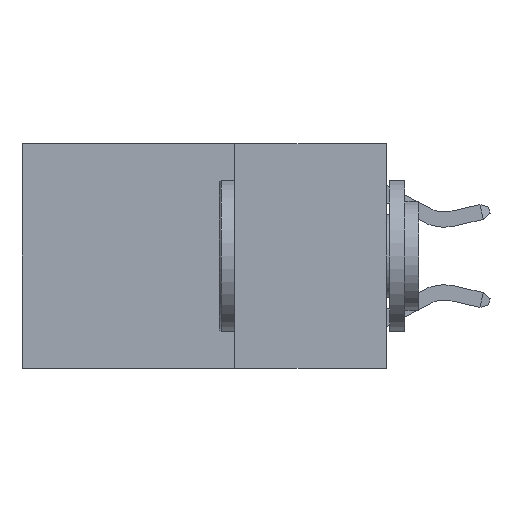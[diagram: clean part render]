
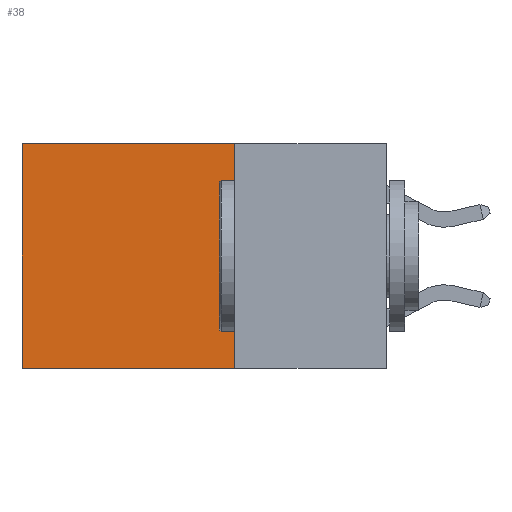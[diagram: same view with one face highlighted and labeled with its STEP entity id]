
A CAD part, left-side view. The second image highlights one B-rep face of the part: STEP entity #38.
In plain terms, the highlighted planar face has unit normal (-1, 0, 0).
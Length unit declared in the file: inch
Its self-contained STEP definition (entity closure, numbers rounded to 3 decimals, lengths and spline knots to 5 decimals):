
#38 = ADVANCED_FACE ( 'NONE', ( #3475 ), #9720, .F. ) ;
#265 = ORIENTED_EDGE ( 'NONE', *, *, #6753, .T. ) ;
#864 = CARTESIAN_POINT ( 'NONE',  ( 0.2625, 0.6, -0.37 ) ) ;
#907 = DIRECTION ( 'NONE',  ( 1., 0., 0. ) ) ;
#1305 = CARTESIAN_POINT ( 'NONE',  ( 0.2625, 0.6, 0. ) ) ;
#1416 = CARTESIAN_POINT ( 'NONE',  ( 0.2625, 0.25, -0.37 ) ) ;
#1434 = DIRECTION ( 'NONE',  ( 0., 1., 0. ) ) ;
#2247 = EDGE_CURVE ( 'NONE', #13000, #3029, #4987, .T. ) ;
#2643 = AXIS2_PLACEMENT_3D ( 'NONE', #9559, #907, #5897 ) ;
#2730 = VERTEX_POINT ( 'NONE', #14551 ) ;
#3029 = VERTEX_POINT ( 'NONE', #864 ) ;
#3475 = FACE_OUTER_BOUND ( 'NONE', #12587, .T. ) ;
#3600 = ORIENTED_EDGE ( 'NONE', *, *, #2247, .T. ) ;
#3756 = LINE ( 'NONE', #4725, #8394 ) ;
#3945 = DIRECTION ( 'NONE',  ( 0., 0., -1. ) ) ;
#4178 = EDGE_CURVE ( 'NONE', #10382, #3029, #5138, .T. ) ;
#4725 = CARTESIAN_POINT ( 'NONE',  ( 0.2625, 0.25, 0. ) ) ;
#4770 = CARTESIAN_POINT ( 'NONE',  ( 0.2625, 0.25, 0. ) ) ;
#4987 = LINE ( 'NONE', #1305, #10707 ) ;
#5094 = DIRECTION ( 'NONE',  ( 0., 1., 0. ) ) ;
#5138 = LINE ( 'NONE', #9843, #6156 ) ;
#5897 = DIRECTION ( 'NONE',  ( 0., 0., -1. ) ) ;
#6156 = VECTOR ( 'NONE', #1434, 39.37008 ) ;
#6753 = EDGE_CURVE ( 'NONE', #2730, #13000, #12289, .T. ) ;
#8155 = ORIENTED_EDGE ( 'NONE', *, *, #13519, .F. ) ;
#8394 = VECTOR ( 'NONE', #14690, 39.37008 ) ;
#9377 = CARTESIAN_POINT ( 'NONE',  ( 0.2625, 0.6, 0. ) ) ;
#9559 = CARTESIAN_POINT ( 'NONE',  ( 0.2625, 0.25, 0. ) ) ;
#9720 = PLANE ( 'NONE',  #2643 ) ;
#9843 = CARTESIAN_POINT ( 'NONE',  ( 0.2625, 0.25, -0.37 ) ) ;
#10382 = VERTEX_POINT ( 'NONE', #1416 ) ;
#10707 = VECTOR ( 'NONE', #3945, 39.37008 ) ;
#12051 = VECTOR ( 'NONE', #5094, 39.37008 ) ;
#12289 = LINE ( 'NONE', #4770, #12051 ) ;
#12587 = EDGE_LOOP ( 'NONE', ( #3600, #13851, #8155, #265 ) ) ;
#13000 = VERTEX_POINT ( 'NONE', #9377 ) ;
#13519 = EDGE_CURVE ( 'NONE', #2730, #10382, #3756, .T. ) ;
#13851 = ORIENTED_EDGE ( 'NONE', *, *, #4178, .F. ) ;
#14551 = CARTESIAN_POINT ( 'NONE',  ( 0.2625, 0.25, 0. ) ) ;
#14690 = DIRECTION ( 'NONE',  ( 0., 0., -1. ) ) ;
